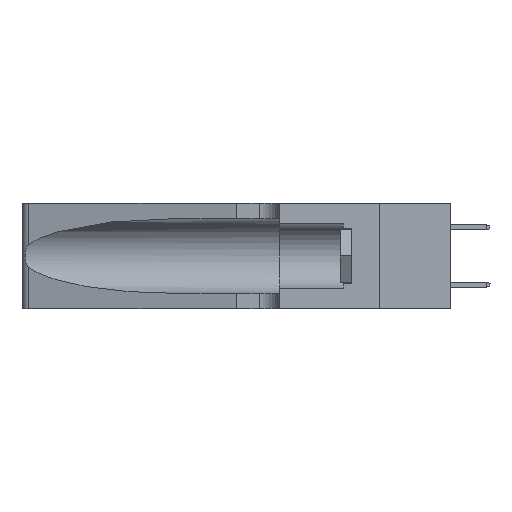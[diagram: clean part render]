
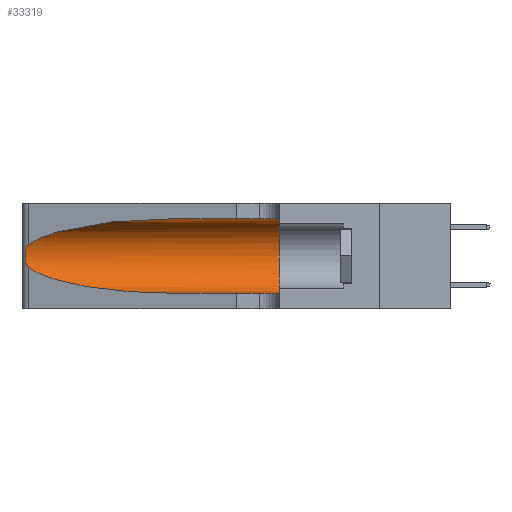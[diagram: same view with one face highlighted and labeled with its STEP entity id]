
A CAD part, left-side view. The second image highlights one B-rep face of the part: STEP entity #33319.
In plain terms, the highlighted cylindrical face has radius 3.308 mm (diameter 6.617 mm), a partial arc.
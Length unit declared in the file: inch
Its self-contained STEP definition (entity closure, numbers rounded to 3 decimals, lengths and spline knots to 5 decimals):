
#214 = CARTESIAN_POINT ( 'NONE',  ( 0.1305, 1.61858, 0.31525 ) ) ;
#550 =( BOUNDED_CURVE ( )  B_SPLINE_CURVE ( 3, ( #33639, #4026, #12984, #36736 ),
 .UNSPECIFIED., .F., .T. ) 
 B_SPLINE_CURVE_WITH_KNOTS ( ( 4, 4 ),
 ( 1.5708, 2.84003 ),
 .UNSPECIFIED. ) 
 CURVE ( )  GEOMETRIC_REPRESENTATION_ITEM ( )  RATIONAL_B_SPLINE_CURVE ( ( 1., 0.87, 0.87, 1. ) ) 
 REPRESENTATION_ITEM ( '' )  );
#2060 = VERTEX_POINT ( 'NONE', #22438 ) ;
#3333 = EDGE_CURVE ( 'NONE', #15257, #35388, #23229, .T. ) ;
#4026 = CARTESIAN_POINT ( 'NONE',  ( 0.18966, 0.96281, 0.31525 ) ) ;
#4034 = DIRECTION ( 'NONE',  ( 0., 1., 0. ) ) ;
#4112 = CARTESIAN_POINT ( 'NONE',  ( 0.26017, 1.23833, 0.17102 ) ) ;
#4886 = CARTESIAN_POINT ( 'NONE',  ( 0.25555, 1.22994, 0.2215 ) ) ;
#5281 = DIRECTION ( 'NONE',  ( 0., 0., -1. ) ) ;
#5986 = ORIENTED_EDGE ( 'NONE', *, *, #3333, .T. ) ;
#6595 = ORIENTED_EDGE ( 'NONE', *, *, #13532, .T. ) ;
#6785 = DIRECTION ( 'NONE',  ( 0., 0., 1. ) ) ;
#7293 = CARTESIAN_POINT ( 'NONE',  ( 0.25487, 1.22718, 0.14631 ) ) ;
#7409 = ORIENTED_EDGE ( 'NONE', *, *, #14226, .T. ) ;
#8018 = CARTESIAN_POINT ( 'NONE',  ( 0.25487, 1.22718, 0.14631 ) ) ;
#8219 = DIRECTION ( 'NONE',  ( 0., -1., 0. ) ) ;
#9496 = EDGE_LOOP ( 'NONE', ( #7409, #27632, #6595, #5986, #31960, #38071 ) ) ;
#10858 = AXIS2_PLACEMENT_3D ( 'NONE', #14239, #8219, #5281 ) ;
#10948 = CARTESIAN_POINT ( 'NONE',  ( 0.26075, 1.23896, 0.19203 ) ) ;
#10957 = FACE_OUTER_BOUND ( 'NONE', #9496, .T. ) ;
#10998 = CARTESIAN_POINT ( 'NONE',  ( 0.18966, 0.96281, 0.05475 ) ) ;
#11166 = CARTESIAN_POINT ( 'NONE',  ( 0.25487, 1.22718, 0.22369 ) ) ;
#11514 = EDGE_CURVE ( 'NONE', #21449, #21231, #30873, .T. ) ;
#12109 = CARTESIAN_POINT ( 'NONE',  ( 0.1305, 0.72297, 0.31525 ) ) ;
#12984 = CARTESIAN_POINT ( 'NONE',  ( 0.2373, 1.15595, 0.28018 ) ) ;
#13468 = CARTESIAN_POINT ( 'NONE',  ( 0.25854, 1.2359, 0.20912 ) ) ;
#13532 = EDGE_CURVE ( 'NONE', #21231, #15257, #28678, .T. ) ;
#13853 = CARTESIAN_POINT ( 'NONE',  ( 0.25856, 1.23593, 0.16098 ) ) ;
#14226 = EDGE_CURVE ( 'NONE', #19524, #21449, #550, .T. ) ;
#14239 = CARTESIAN_POINT ( 'NONE',  ( 0.1305, 1.61858, 0.185 ) ) ;
#14379 = CARTESIAN_POINT ( 'NONE',  ( 0.1305, 0.72297, 0.05475 ) ) ;
#15257 = VERTEX_POINT ( 'NONE', #14379 ) ;
#15624 = DIRECTION ( 'NONE',  ( 0., -1., 0. ) ) ;
#16766 = CARTESIAN_POINT ( 'NONE',  ( 0.25787, 1.23484, 0.2124 ) ) ;
#18957 = CARTESIAN_POINT ( 'NONE',  ( 0.26018, 1.23835, 0.19895 ) ) ;
#19140 = CARTESIAN_POINT ( 'NONE',  ( 0.25487, 1.22718, 0.22369 ) ) ;
#19524 = VERTEX_POINT ( 'NONE', #12109 ) ;
#19575 = CARTESIAN_POINT ( 'NONE',  ( 0.25487, 1.22718, 0.14631 ) ) ;
#21231 = VERTEX_POINT ( 'NONE', #7293 ) ;
#21342 = CARTESIAN_POINT ( 'NONE',  ( 0.1305, 0.35, 0.05475 ) ) ;
#21449 = VERTEX_POINT ( 'NONE', #11166 ) ;
#21943 = CIRCLE ( 'NONE', #26276, 0.13025 ) ;
#22438 = CARTESIAN_POINT ( 'NONE',  ( 0.1305, 0.35, 0.31525 ) ) ;
#23229 = LINE ( 'NONE', #35051, #29575 ) ;
#23555 = EDGE_CURVE ( 'NONE', #2060, #35388, #21943, .T. ) ;
#26276 = AXIS2_PLACEMENT_3D ( 'NONE', #30178, #4034, #6785 ) ;
#26714 = CARTESIAN_POINT ( 'NONE',  ( 0.25789, 1.23486, 0.15765 ) ) ;
#27374 = EDGE_CURVE ( 'NONE', #19524, #2060, #30429, .T. ) ;
#27389 = VECTOR ( 'NONE', #15624, 39.37008 ) ;
#27632 = ORIENTED_EDGE ( 'NONE', *, *, #11514, .T. ) ;
#28656 = CARTESIAN_POINT ( 'NONE',  ( 0.26075, 1.23896, 0.178 ) ) ;
#28678 =( BOUNDED_CURVE ( )  B_SPLINE_CURVE ( 3, ( #19575, #34340, #10998, #28711 ),
 .UNSPECIFIED., .F., .T. ) 
 B_SPLINE_CURVE_WITH_KNOTS ( ( 4, 4 ),
 ( 3.44316, 4.71239 ),
 .UNSPECIFIED. ) 
 CURVE ( )  GEOMETRIC_REPRESENTATION_ITEM ( )  RATIONAL_B_SPLINE_CURVE ( ( 1., 0.87, 0.87, 1. ) ) 
 REPRESENTATION_ITEM ( '' )  );
#28711 = CARTESIAN_POINT ( 'NONE',  ( 0.1305, 0.72297, 0.05475 ) ) ;
#29575 = VECTOR ( 'NONE', #38360, 39.37008 ) ;
#29635 = CARTESIAN_POINT ( 'NONE',  ( 0.25555, 1.22993, 0.14849 ) ) ;
#30178 = CARTESIAN_POINT ( 'NONE',  ( 0.1305, 0.35, 0.185 ) ) ;
#30429 = LINE ( 'NONE', #214, #27389 ) ;
#30873 = B_SPLINE_CURVE_WITH_KNOTS ( 'NONE', 3,
 ( #19140, #4886, #31015, #16766, #13468, #18957, #10948, #28656, #4112, #13853, #26714, #34840, #29635, #8018 ),
 .UNSPECIFIED., .F., .F.,
 ( 4, 2, 2, 2, 2, 2, 4 ),
 ( 0., 0.00027, 0.00053, 0.00107, 0.0016, 0.00187, 0.00214 ),
 .UNSPECIFIED. ) ;
#31015 = CARTESIAN_POINT ( 'NONE',  ( 0.25639, 1.23184, 0.21858 ) ) ;
#31960 = ORIENTED_EDGE ( 'NONE', *, *, #23555, .F. ) ;
#33319 = ADVANCED_FACE ( 'NONE', ( #10957 ), #37214, .F. ) ;
#33639 = CARTESIAN_POINT ( 'NONE',  ( 0.1305, 0.72297, 0.31525 ) ) ;
#34340 = CARTESIAN_POINT ( 'NONE',  ( 0.2373, 1.15595, 0.08982 ) ) ;
#34840 = CARTESIAN_POINT ( 'NONE',  ( 0.25639, 1.23186, 0.15144 ) ) ;
#35051 = CARTESIAN_POINT ( 'NONE',  ( 0.1305, 1.61858, 0.05475 ) ) ;
#35388 = VERTEX_POINT ( 'NONE', #21342 ) ;
#36736 = CARTESIAN_POINT ( 'NONE',  ( 0.25487, 1.22718, 0.22369 ) ) ;
#37214 = CYLINDRICAL_SURFACE ( 'NONE', #10858, 0.13025 ) ;
#38071 = ORIENTED_EDGE ( 'NONE', *, *, #27374, .F. ) ;
#38360 = DIRECTION ( 'NONE',  ( 0., -1., 0. ) ) ;
